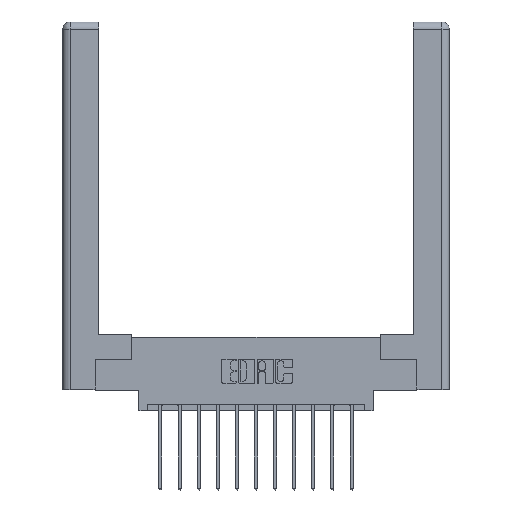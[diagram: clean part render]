
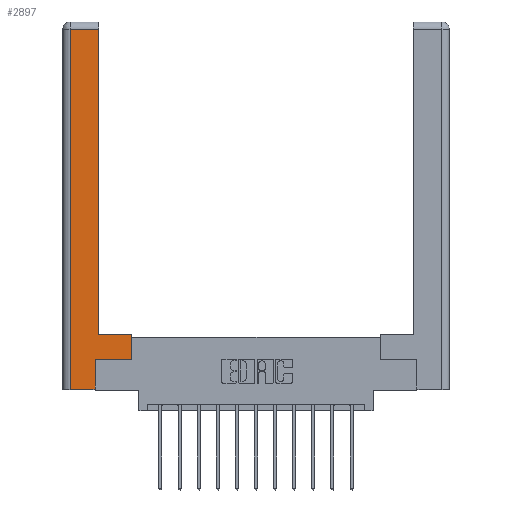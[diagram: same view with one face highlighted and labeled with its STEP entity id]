
A CAD part, top view. The second image highlights one B-rep face of the part: STEP entity #2897.
In plain terms, the highlighted planar face has unit normal (0, 0, 1).
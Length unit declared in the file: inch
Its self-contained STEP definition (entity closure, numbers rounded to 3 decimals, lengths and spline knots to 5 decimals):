
#55 = LINE ( 'NONE', #233, #13425 ) ;
#65 = DIRECTION ( 'NONE',  ( 0., 1., 0. ) ) ;
#142 = CARTESIAN_POINT ( 'NONE',  ( 0.265, 0.245, 0. ) ) ;
#233 = CARTESIAN_POINT ( 'NONE',  ( 0.265, 0., 0. ) ) ;
#426 = ORIENTED_EDGE ( 'NONE', *, *, #6659, .T. ) ;
#479 = LINE ( 'NONE', #4798, #9935 ) ;
#726 = CARTESIAN_POINT ( 'NONE',  ( 0., 0., 0. ) ) ;
#805 = LINE ( 'NONE', #13936, #9525 ) ;
#888 = CARTESIAN_POINT ( 'NONE',  ( 0.295, 0.45, 0. ) ) ;
#925 = CARTESIAN_POINT ( 'NONE',  ( 0.295, 0.45, 0. ) ) ;
#1224 = DIRECTION ( 'NONE',  ( 0., -1., 0. ) ) ;
#1258 = DIRECTION ( 'NONE',  ( -1., 0., 0. ) ) ;
#2409 = EDGE_CURVE ( 'NONE', #8227, #14583, #10842, .T. ) ;
#2525 = CARTESIAN_POINT ( 'NONE',  ( 0.0615, 0., 0. ) ) ;
#2897 = ADVANCED_FACE ( 'NONE', ( #11574 ), #13670, .F. ) ;
#3326 = DIRECTION ( 'NONE',  ( 1., 0., 0. ) ) ;
#4097 = CARTESIAN_POINT ( 'NONE',  ( 0.295, 2.94, 0. ) ) ;
#4264 = EDGE_CURVE ( 'NONE', #7390, #10992, #14795, .T. ) ;
#4413 = VECTOR ( 'NONE', #1224, 39.37008 ) ;
#4798 = CARTESIAN_POINT ( 'NONE',  ( 0.265, 0.245, 0. ) ) ;
#4954 = ORIENTED_EDGE ( 'NONE', *, *, #2409, .T. ) ;
#5274 = ORIENTED_EDGE ( 'NONE', *, *, #13586, .T. ) ;
#5574 = CARTESIAN_POINT ( 'NONE',  ( 0.295, 3., 0. ) ) ;
#6069 = DIRECTION ( 'NONE',  ( 1., 0., 0. ) ) ;
#6170 = VECTOR ( 'NONE', #7826, 39.37008 ) ;
#6659 = EDGE_CURVE ( 'NONE', #14583, #10961, #55, .T. ) ;
#6774 = VERTEX_POINT ( 'NONE', #4097 ) ;
#6854 = AXIS2_PLACEMENT_3D ( 'NONE', #726, #12874, #12652 ) ;
#7274 = LINE ( 'NONE', #888, #12212 ) ;
#7389 = EDGE_CURVE ( 'NONE', #15350, #7390, #805, .T. ) ;
#7390 = VERTEX_POINT ( 'NONE', #15101 ) ;
#7451 = DIRECTION ( 'NONE',  ( 0., 1., 0. ) ) ;
#7826 = DIRECTION ( 'NONE',  ( -1., 0., 0. ) ) ;
#8026 = VECTOR ( 'NONE', #65, 39.37008 ) ;
#8227 = VERTEX_POINT ( 'NONE', #10331 ) ;
#8421 = CARTESIAN_POINT ( 'NONE',  ( 0.265, 0., 0. ) ) ;
#8572 = EDGE_CURVE ( 'NONE', #6774, #8227, #12826, .T. ) ;
#8663 = EDGE_CURVE ( 'NONE', #12445, #6774, #15033, .T. ) ;
#8808 = ORIENTED_EDGE ( 'NONE', *, *, #11707, .T. ) ;
#9319 = EDGE_LOOP ( 'NONE', ( #10197, #14358, #4954, #426, #5274, #9842, #14641, #8808 ) ) ;
#9525 = VECTOR ( 'NONE', #3326, 39.37008 ) ;
#9842 = ORIENTED_EDGE ( 'NONE', *, *, #7389, .T. ) ;
#9935 = VECTOR ( 'NONE', #13028, 39.37008 ) ;
#10197 = ORIENTED_EDGE ( 'NONE', *, *, #8663, .T. ) ;
#10331 = CARTESIAN_POINT ( 'NONE',  ( 0.0615, 2.94, 0. ) ) ;
#10842 = LINE ( 'NONE', #13053, #4413 ) ;
#10961 = VERTEX_POINT ( 'NONE', #8421 ) ;
#10992 = VERTEX_POINT ( 'NONE', #12978 ) ;
#11084 = VECTOR ( 'NONE', #7451, 39.37008 ) ;
#11574 = FACE_OUTER_BOUND ( 'NONE', #9319, .T. ) ;
#11707 = EDGE_CURVE ( 'NONE', #10992, #12445, #7274, .T. ) ;
#11774 = CARTESIAN_POINT ( 'NONE',  ( 0.0615, 2.94, 0. ) ) ;
#12212 = VECTOR ( 'NONE', #1258, 39.37008 ) ;
#12445 = VERTEX_POINT ( 'NONE', #925 ) ;
#12652 = DIRECTION ( 'NONE',  ( -1., 0., 0. ) ) ;
#12826 = LINE ( 'NONE', #11774, #6170 ) ;
#12874 = DIRECTION ( 'NONE',  ( 0., 0., -1. ) ) ;
#12978 = CARTESIAN_POINT ( 'NONE',  ( 0.565, 0.45, 0. ) ) ;
#13028 = DIRECTION ( 'NONE',  ( 0., 1., 0. ) ) ;
#13053 = CARTESIAN_POINT ( 'NONE',  ( 0.0615, 0., 0. ) ) ;
#13425 = VECTOR ( 'NONE', #6069, 39.37008 ) ;
#13586 = EDGE_CURVE ( 'NONE', #10961, #15350, #479, .T. ) ;
#13670 = PLANE ( 'NONE',  #6854 ) ;
#13936 = CARTESIAN_POINT ( 'NONE',  ( 0.565, 0.245, 0. ) ) ;
#14358 = ORIENTED_EDGE ( 'NONE', *, *, #8572, .T. ) ;
#14421 = CARTESIAN_POINT ( 'NONE',  ( 0.565, 0.45, 0. ) ) ;
#14583 = VERTEX_POINT ( 'NONE', #2525 ) ;
#14641 = ORIENTED_EDGE ( 'NONE', *, *, #4264, .T. ) ;
#14795 = LINE ( 'NONE', #14421, #11084 ) ;
#15033 = LINE ( 'NONE', #5574, #8026 ) ;
#15101 = CARTESIAN_POINT ( 'NONE',  ( 0.565, 0.245, 0. ) ) ;
#15350 = VERTEX_POINT ( 'NONE', #142 ) ;
